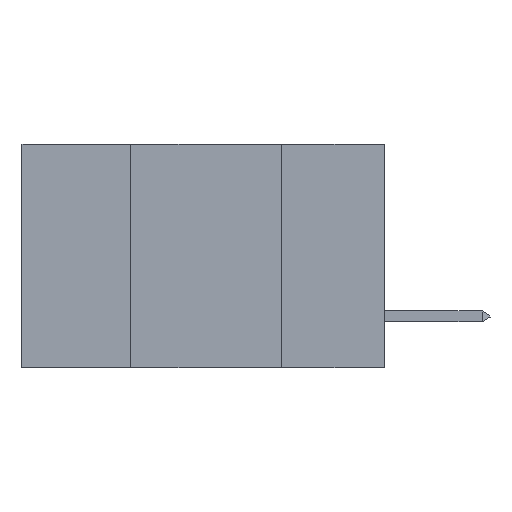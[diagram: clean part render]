
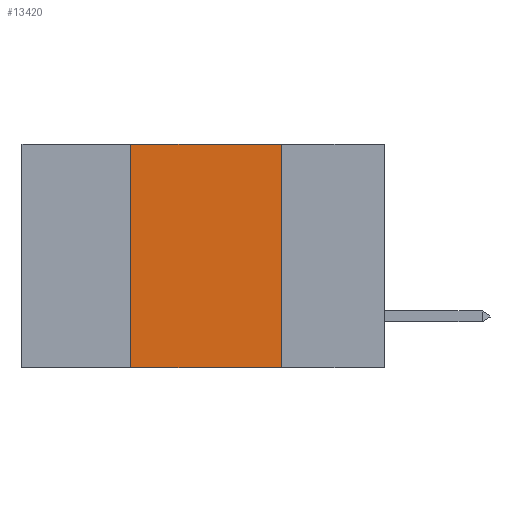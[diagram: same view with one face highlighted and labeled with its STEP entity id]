
A CAD part, left-side view. The second image highlights one B-rep face of the part: STEP entity #13420.
In plain terms, the highlighted planar face has unit normal (-1, 0, 0).
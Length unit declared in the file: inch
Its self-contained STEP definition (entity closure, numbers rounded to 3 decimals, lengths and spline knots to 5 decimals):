
#1117 = EDGE_CURVE ( 'NONE', #19169, #12319, #17448, .T. ) ;
#2040 = EDGE_CURVE ( 'NONE', #20327, #3621, #20012, .T. ) ;
#2637 = ORIENTED_EDGE ( 'NONE', *, *, #26848, .T. ) ;
#2957 = CARTESIAN_POINT ( 'NONE',  ( 0., 0.17, -0.37 ) ) ;
#3621 = VERTEX_POINT ( 'NONE', #17846 ) ;
#4040 = DIRECTION ( 'NONE',  ( 0., -1., 0. ) ) ;
#5676 = VECTOR ( 'NONE', #4040, 39.37008 ) ;
#6740 = FACE_OUTER_BOUND ( 'NONE', #20001, .T. ) ;
#6967 = DIRECTION ( 'NONE',  ( 0., -1., 0. ) ) ;
#8997 = CARTESIAN_POINT ( 'NONE',  ( 0., 0.6, -0.37 ) ) ;
#9033 = VECTOR ( 'NONE', #24784, 39.37008 ) ;
#9042 = CARTESIAN_POINT ( 'NONE',  ( 0., 0.6, 0. ) ) ;
#11185 = LINE ( 'NONE', #12546, #5676 ) ;
#11342 = ORIENTED_EDGE ( 'NONE', *, *, #2040, .F. ) ;
#12319 = VERTEX_POINT ( 'NONE', #2957 ) ;
#12546 = CARTESIAN_POINT ( 'NONE',  ( 0., 0.6, 0. ) ) ;
#12911 = PLANE ( 'NONE',  #26345 ) ;
#13420 = ADVANCED_FACE ( 'NONE', ( #6740 ), #12911, .F. ) ;
#15553 = DIRECTION ( 'NONE',  ( 1., 0., 0. ) ) ;
#15741 = VECTOR ( 'NONE', #6967, 39.37008 ) ;
#15946 = CARTESIAN_POINT ( 'NONE',  ( 0., 0.42, 0. ) ) ;
#16934 = CARTESIAN_POINT ( 'NONE',  ( 0., 0.42, -0.37 ) ) ;
#17448 = LINE ( 'NONE', #20368, #9033 ) ;
#17846 = CARTESIAN_POINT ( 'NONE',  ( 0., 0.42, 0. ) ) ;
#18012 = DIRECTION ( 'NONE',  ( 0., 0., 1. ) ) ;
#18731 = CARTESIAN_POINT ( 'NONE',  ( 0., 0.17, 0. ) ) ;
#18984 = LINE ( 'NONE', #8997, #15741 ) ;
#19169 = VERTEX_POINT ( 'NONE', #18731 ) ;
#19183 = EDGE_CURVE ( 'NONE', #3621, #19169, #11185, .T. ) ;
#20001 = EDGE_LOOP ( 'NONE', ( #23385, #25603, #11342, #2637 ) ) ;
#20012 = LINE ( 'NONE', #15946, #24874 ) ;
#20327 = VERTEX_POINT ( 'NONE', #16934 ) ;
#20368 = CARTESIAN_POINT ( 'NONE',  ( 0., 0.17, 0. ) ) ;
#23385 = ORIENTED_EDGE ( 'NONE', *, *, #1117, .F. ) ;
#23802 = DIRECTION ( 'NONE',  ( 0., 0., -1. ) ) ;
#24784 = DIRECTION ( 'NONE',  ( 0., 0., -1. ) ) ;
#24874 = VECTOR ( 'NONE', #18012, 39.37008 ) ;
#25603 = ORIENTED_EDGE ( 'NONE', *, *, #19183, .F. ) ;
#26345 = AXIS2_PLACEMENT_3D ( 'NONE', #9042, #15553, #23802 ) ;
#26848 = EDGE_CURVE ( 'NONE', #20327, #12319, #18984, .T. ) ;
